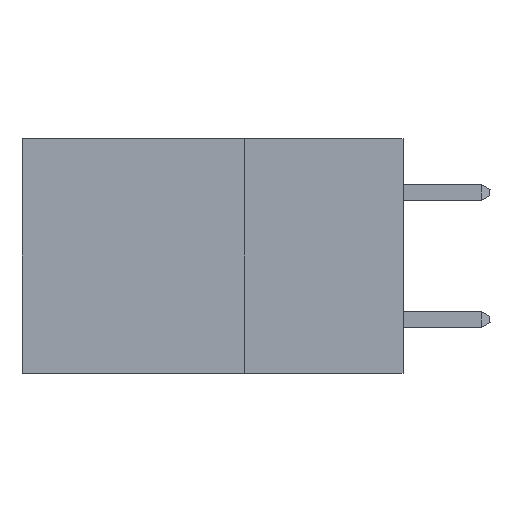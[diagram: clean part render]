
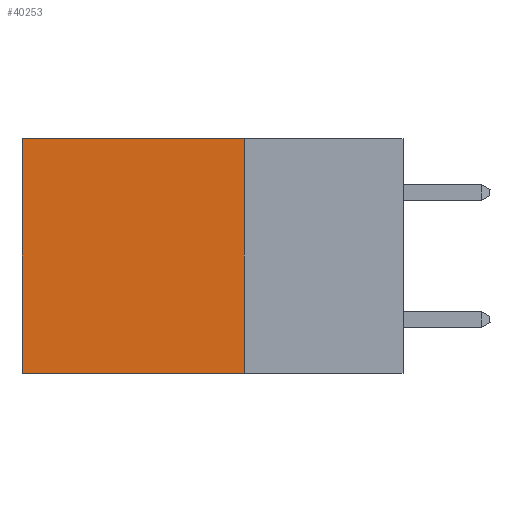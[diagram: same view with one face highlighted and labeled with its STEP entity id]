
A CAD part, left-side view. The second image highlights one B-rep face of the part: STEP entity #40253.
In plain terms, the highlighted planar face has unit normal (-1, 0, 0).
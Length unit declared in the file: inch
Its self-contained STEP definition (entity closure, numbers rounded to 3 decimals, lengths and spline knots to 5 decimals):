
#724 = VECTOR ( 'NONE', #31366, 39.37008 ) ;
#770 = CARTESIAN_POINT ( 'NONE',  ( 0.2875, 0.25, 0. ) ) ;
#1621 = CARTESIAN_POINT ( 'NONE',  ( 0.2875, 0.25, 0. ) ) ;
#2824 = CARTESIAN_POINT ( 'NONE',  ( 0.2875, 0.6, -0.37 ) ) ;
#3082 = LINE ( 'NONE', #770, #23082 ) ;
#8530 = VERTEX_POINT ( 'NONE', #2824 ) ;
#9464 = ORIENTED_EDGE ( 'NONE', *, *, #19134, .T. ) ;
#11954 = VECTOR ( 'NONE', #16601, 39.37008 ) ;
#12564 = CARTESIAN_POINT ( 'NONE',  ( 0.2875, 0.25, -0.37 ) ) ;
#14587 = VECTOR ( 'NONE', #35573, 39.37008 ) ;
#14984 = CARTESIAN_POINT ( 'NONE',  ( 0.2875, 0.25, -0.37 ) ) ;
#15643 = EDGE_CURVE ( 'NONE', #46133, #31623, #3082, .T. ) ;
#15645 = PLANE ( 'NONE',  #30512 ) ;
#16601 = DIRECTION ( 'NONE',  ( 0., 0., -1. ) ) ;
#18522 = DIRECTION ( 'NONE',  ( 0., 1., 0. ) ) ;
#19134 = EDGE_CURVE ( 'NONE', #31623, #8530, #43920, .T. ) ;
#21839 = FACE_OUTER_BOUND ( 'NONE', #21892, .T. ) ;
#21865 = CARTESIAN_POINT ( 'NONE',  ( 0.2875, 0.25, 0. ) ) ;
#21892 = EDGE_LOOP ( 'NONE', ( #9464, #36719, #29887, #39726 ) ) ;
#23082 = VECTOR ( 'NONE', #18522, 39.37008 ) ;
#27430 = EDGE_CURVE ( 'NONE', #47203, #8530, #38946, .T. ) ;
#29194 = DIRECTION ( 'NONE',  ( 0., 0., -1. ) ) ;
#29887 = ORIENTED_EDGE ( 'NONE', *, *, #31086, .F. ) ;
#30512 = AXIS2_PLACEMENT_3D ( 'NONE', #21865, #47259, #29194 ) ;
#30744 = CARTESIAN_POINT ( 'NONE',  ( 0.2875, 0.6, 0. ) ) ;
#31086 = EDGE_CURVE ( 'NONE', #46133, #47203, #35067, .T. ) ;
#31366 = DIRECTION ( 'NONE',  ( 0., 1., 0. ) ) ;
#31623 = VERTEX_POINT ( 'NONE', #39459 ) ;
#35067 = LINE ( 'NONE', #46486, #14587 ) ;
#35573 = DIRECTION ( 'NONE',  ( 0., 0., -1. ) ) ;
#36719 = ORIENTED_EDGE ( 'NONE', *, *, #27430, .F. ) ;
#38946 = LINE ( 'NONE', #12564, #724 ) ;
#39459 = CARTESIAN_POINT ( 'NONE',  ( 0.2875, 0.6, 0. ) ) ;
#39726 = ORIENTED_EDGE ( 'NONE', *, *, #15643, .T. ) ;
#40253 = ADVANCED_FACE ( 'NONE', ( #21839 ), #15645, .F. ) ;
#43920 = LINE ( 'NONE', #30744, #11954 ) ;
#46133 = VERTEX_POINT ( 'NONE', #1621 ) ;
#46486 = CARTESIAN_POINT ( 'NONE',  ( 0.2875, 0.25, 0. ) ) ;
#47203 = VERTEX_POINT ( 'NONE', #14984 ) ;
#47259 = DIRECTION ( 'NONE',  ( 1., 0., 0. ) ) ;
